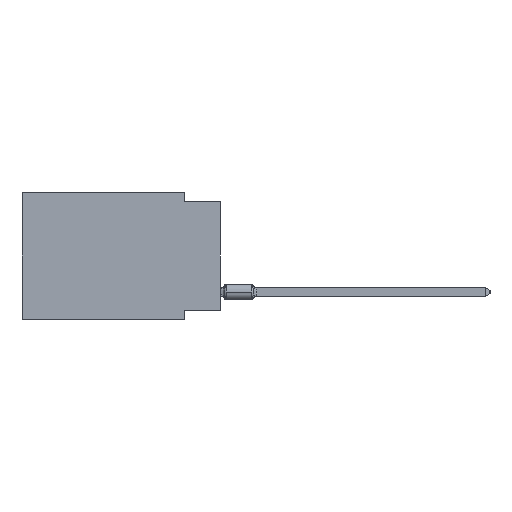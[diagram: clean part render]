
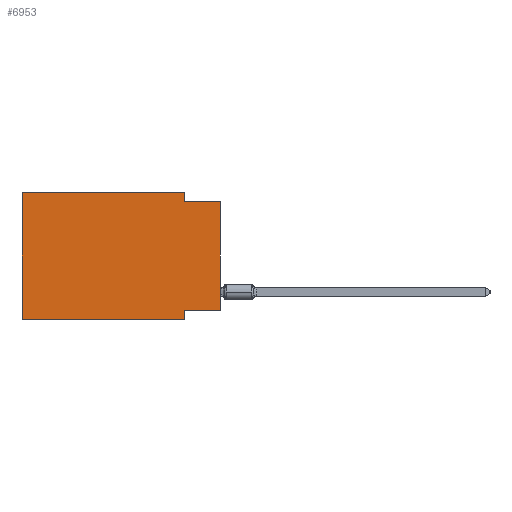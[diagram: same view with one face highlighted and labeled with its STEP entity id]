
A CAD part, left-side view. The second image highlights one B-rep face of the part: STEP entity #6953.
In plain terms, the highlighted planar face has unit normal (-1, 0, 0).
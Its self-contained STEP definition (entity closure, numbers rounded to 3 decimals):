
#746 = LINE ( 'NONE', #6038, #24364 ) ;
#943 = LINE ( 'NONE', #15132, #5036 ) ;
#1287 = ORIENTED_EDGE ( 'NONE', *, *, #22459, .T. ) ;
#1794 = EDGE_CURVE ( 'NONE', #18026, #11206, #12615, .T. ) ;
#2128 = ORIENTED_EDGE ( 'NONE', *, *, #24853, .F. ) ;
#2358 = EDGE_CURVE ( 'NONE', #27625, #18026, #20949, .T. ) ;
#3376 = EDGE_CURVE ( 'NONE', #19621, #34539, #746, .T. ) ;
#3751 = DIRECTION ( 'NONE',  ( 0., 0., 1. ) ) ;
#5036 = VECTOR ( 'NONE', #20462, 1000. ) ;
#5467 = CARTESIAN_POINT ( 'NONE',  ( 0., 2.54, -8.255 ) ) ;
#6038 = CARTESIAN_POINT ( 'NONE',  ( 0., 0., 0. ) ) ;
#6152 = CARTESIAN_POINT ( 'NONE',  ( 0., 2.54, -8.89 ) ) ;
#6363 = LINE ( 'NONE', #11852, #33618 ) ;
#6469 = VERTEX_POINT ( 'NONE', #5467 ) ;
#6953 = ADVANCED_FACE ( 'NONE', ( #11255 ), #21767, .F. ) ;
#7775 = DIRECTION ( 'NONE',  ( 0., -1., 0. ) ) ;
#9246 = CARTESIAN_POINT ( 'NONE',  ( 0., 0., -0.635 ) ) ;
#10332 = ORIENTED_EDGE ( 'NONE', *, *, #29205, .F. ) ;
#11206 = VERTEX_POINT ( 'NONE', #15638 ) ;
#11255 = FACE_OUTER_BOUND ( 'NONE', #15307, .T. ) ;
#11495 = VECTOR ( 'NONE', #15096, 1000. ) ;
#11837 = ORIENTED_EDGE ( 'NONE', *, *, #15894, .F. ) ;
#11852 = CARTESIAN_POINT ( 'NONE',  ( 0., 0., -8.255 ) ) ;
#12615 = LINE ( 'NONE', #19577, #34951 ) ;
#12812 = CARTESIAN_POINT ( 'NONE',  ( 0., 13.97, -8.89 ) ) ;
#14046 = ORIENTED_EDGE ( 'NONE', *, *, #34987, .F. ) ;
#14734 = LINE ( 'NONE', #30893, #25002 ) ;
#15096 = DIRECTION ( 'NONE',  ( 0., -1., 0. ) ) ;
#15132 = CARTESIAN_POINT ( 'NONE',  ( 0., 2.54, -8.89 ) ) ;
#15307 = EDGE_LOOP ( 'NONE', ( #16873, #11837, #31739, #29820, #14046, #1287, #10332, #2128 ) ) ;
#15638 = CARTESIAN_POINT ( 'NONE',  ( 0., 2.54, -0.635 ) ) ;
#15894 = EDGE_CURVE ( 'NONE', #11206, #34539, #14734, .T. ) ;
#16873 = ORIENTED_EDGE ( 'NONE', *, *, #3376, .T. ) ;
#17229 = DIRECTION ( 'NONE',  ( 0., -1., 0. ) ) ;
#17860 = CARTESIAN_POINT ( 'NONE',  ( 0., 13.97, 0. ) ) ;
#18016 = AXIS2_PLACEMENT_3D ( 'NONE', #21919, #27425, #33266 ) ;
#18026 = VERTEX_POINT ( 'NONE', #21173 ) ;
#18773 = VECTOR ( 'NONE', #7775, 1000. ) ;
#19382 = VECTOR ( 'NONE', #28680, 1000. ) ;
#19577 = CARTESIAN_POINT ( 'NONE',  ( 0., 2.54, 0. ) ) ;
#19621 = VERTEX_POINT ( 'NONE', #29266 ) ;
#20462 = DIRECTION ( 'NONE',  ( 0., 0., -1. ) ) ;
#20949 = LINE ( 'NONE', #31584, #11495 ) ;
#21173 = CARTESIAN_POINT ( 'NONE',  ( 0., 2.54, 0. ) ) ;
#21767 = PLANE ( 'NONE',  #18016 ) ;
#21919 = CARTESIAN_POINT ( 'NONE',  ( 0., 13.97, 0. ) ) ;
#22459 = EDGE_CURVE ( 'NONE', #27280, #22619, #23953, .T. ) ;
#22619 = VERTEX_POINT ( 'NONE', #6152 ) ;
#22683 = DIRECTION ( 'NONE',  ( 0., 1., 0. ) ) ;
#23953 = LINE ( 'NONE', #32102, #18773 ) ;
#24090 = CARTESIAN_POINT ( 'NONE',  ( 0., 13.97, 0. ) ) ;
#24364 = VECTOR ( 'NONE', #3751, 1000. ) ;
#24853 = EDGE_CURVE ( 'NONE', #19621, #6469, #6363, .T. ) ;
#25002 = VECTOR ( 'NONE', #17229, 1000. ) ;
#27280 = VERTEX_POINT ( 'NONE', #12812 ) ;
#27425 = DIRECTION ( 'NONE',  ( 1., 0., 0. ) ) ;
#27625 = VERTEX_POINT ( 'NONE', #24090 ) ;
#27731 = DIRECTION ( 'NONE',  ( 0., 0., -1. ) ) ;
#28680 = DIRECTION ( 'NONE',  ( 0., 0., 1. ) ) ;
#29205 = EDGE_CURVE ( 'NONE', #6469, #22619, #943, .T. ) ;
#29266 = CARTESIAN_POINT ( 'NONE',  ( 0., 0., -8.255 ) ) ;
#29820 = ORIENTED_EDGE ( 'NONE', *, *, #2358, .F. ) ;
#30893 = CARTESIAN_POINT ( 'NONE',  ( 0., 0., -0.635 ) ) ;
#31353 = LINE ( 'NONE', #17860, #19382 ) ;
#31584 = CARTESIAN_POINT ( 'NONE',  ( 0., 13.97, 0. ) ) ;
#31739 = ORIENTED_EDGE ( 'NONE', *, *, #1794, .F. ) ;
#32102 = CARTESIAN_POINT ( 'NONE',  ( 0., 13.97, -8.89 ) ) ;
#33266 = DIRECTION ( 'NONE',  ( 0., 0., -1. ) ) ;
#33618 = VECTOR ( 'NONE', #22683, 1000. ) ;
#34539 = VERTEX_POINT ( 'NONE', #9246 ) ;
#34951 = VECTOR ( 'NONE', #27731, 1000. ) ;
#34987 = EDGE_CURVE ( 'NONE', #27280, #27625, #31353, .T. ) ;
